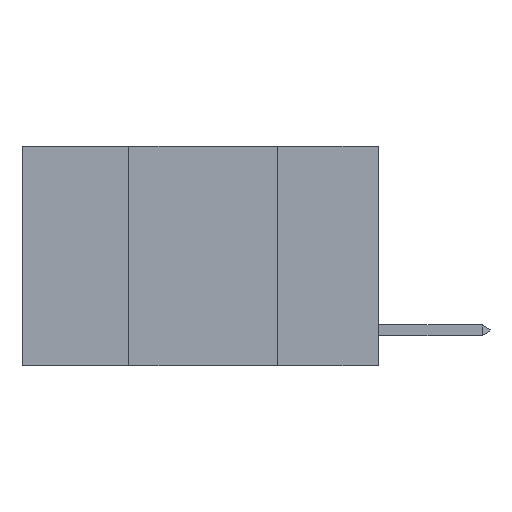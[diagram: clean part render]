
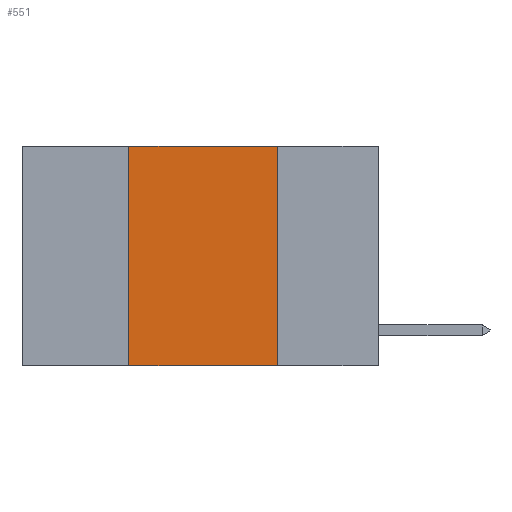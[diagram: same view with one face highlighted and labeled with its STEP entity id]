
A CAD part, left-side view. The second image highlights one B-rep face of the part: STEP entity #551.
In plain terms, the highlighted planar face has unit normal (-1, 0, 0).
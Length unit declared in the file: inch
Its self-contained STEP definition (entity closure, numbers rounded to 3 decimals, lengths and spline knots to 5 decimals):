
#551 = ADVANCED_FACE ( 'NONE', ( #7085 ), #12933, .F. ) ;
#2462 = CARTESIAN_POINT ( 'NONE',  ( 0., 0.6, -0.37 ) ) ;
#2560 = CARTESIAN_POINT ( 'NONE',  ( 0., 0.6, 0. ) ) ;
#3705 = VERTEX_POINT ( 'NONE', #14786 ) ;
#3812 = ORIENTED_EDGE ( 'NONE', *, *, #12539, .F. ) ;
#3917 = CARTESIAN_POINT ( 'NONE',  ( 0., 0.17, 0. ) ) ;
#4333 = CARTESIAN_POINT ( 'NONE',  ( 0., 0.42, -0.37 ) ) ;
#4675 = VERTEX_POINT ( 'NONE', #6537 ) ;
#5669 = DIRECTION ( 'NONE',  ( 0., -1., 0. ) ) ;
#6491 = CARTESIAN_POINT ( 'NONE',  ( 0., 0.42, 0. ) ) ;
#6537 = CARTESIAN_POINT ( 'NONE',  ( 0., 0.17, -0.37 ) ) ;
#7085 = FACE_OUTER_BOUND ( 'NONE', #15829, .T. ) ;
#7266 = ORIENTED_EDGE ( 'NONE', *, *, #13675, .F. ) ;
#7380 = CARTESIAN_POINT ( 'NONE',  ( 0., 0.6, 0. ) ) ;
#7608 = VECTOR ( 'NONE', #21728, 39.37008 ) ;
#7871 = CARTESIAN_POINT ( 'NONE',  ( 0., 0.17, 0. ) ) ;
#8224 = VERTEX_POINT ( 'NONE', #7871 ) ;
#9046 = DIRECTION ( 'NONE',  ( 1., 0., 0. ) ) ;
#9241 = VECTOR ( 'NONE', #15830, 39.37008 ) ;
#9245 = DIRECTION ( 'NONE',  ( 0., 0., -1. ) ) ;
#11213 = EDGE_CURVE ( 'NONE', #3705, #8224, #14332, .T. ) ;
#11818 = LINE ( 'NONE', #2462, #20221 ) ;
#12139 = LINE ( 'NONE', #6491, #7608 ) ;
#12539 = EDGE_CURVE ( 'NONE', #8224, #4675, #13745, .T. ) ;
#12933 = PLANE ( 'NONE',  #19484 ) ;
#13675 = EDGE_CURVE ( 'NONE', #18778, #3705, #12139, .T. ) ;
#13745 = LINE ( 'NONE', #3917, #9241 ) ;
#13804 = VECTOR ( 'NONE', #5669, 39.37008 ) ;
#14332 = LINE ( 'NONE', #7380, #13804 ) ;
#14786 = CARTESIAN_POINT ( 'NONE',  ( 0., 0.42, 0. ) ) ;
#14789 = EDGE_CURVE ( 'NONE', #18778, #4675, #11818, .T. ) ;
#15829 = EDGE_LOOP ( 'NONE', ( #3812, #16728, #7266, #16927 ) ) ;
#15830 = DIRECTION ( 'NONE',  ( 0., 0., -1. ) ) ;
#16728 = ORIENTED_EDGE ( 'NONE', *, *, #11213, .F. ) ;
#16927 = ORIENTED_EDGE ( 'NONE', *, *, #14789, .T. ) ;
#18778 = VERTEX_POINT ( 'NONE', #4333 ) ;
#19484 = AXIS2_PLACEMENT_3D ( 'NONE', #2560, #9046, #9245 ) ;
#20221 = VECTOR ( 'NONE', #21235, 39.37008 ) ;
#21235 = DIRECTION ( 'NONE',  ( 0., -1., 0. ) ) ;
#21728 = DIRECTION ( 'NONE',  ( 0., 0., 1. ) ) ;
